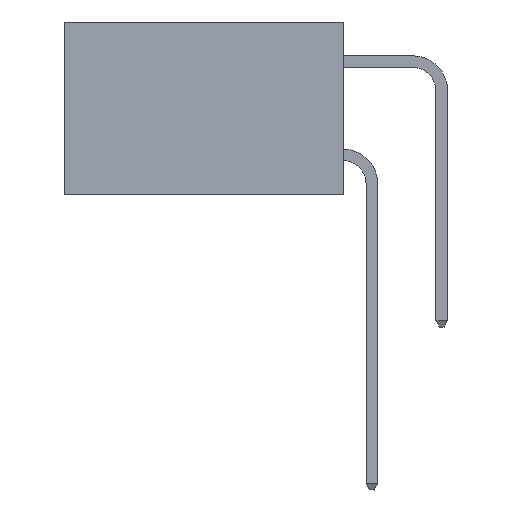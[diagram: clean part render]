
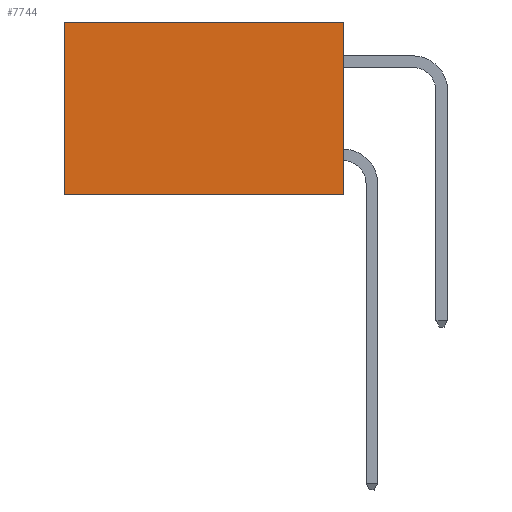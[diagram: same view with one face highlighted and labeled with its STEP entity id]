
A CAD part, left-side view. The second image highlights one B-rep face of the part: STEP entity #7744.
In plain terms, the highlighted planar face has unit normal (-1, 0, 0).
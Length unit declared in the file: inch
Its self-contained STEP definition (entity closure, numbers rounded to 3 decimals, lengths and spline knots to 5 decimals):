
#1168 = DIRECTION ( 'NONE',  ( 0., 1., 0. ) ) ;
#1582 = ORIENTED_EDGE ( 'NONE', *, *, #8854, .F. ) ;
#1912 = DIRECTION ( 'NONE',  ( 0., 0., -1. ) ) ;
#1956 = DIRECTION ( 'NONE',  ( 1., 0., 0. ) ) ;
#1972 = CARTESIAN_POINT ( 'NONE',  ( 0.298, 0., 0. ) ) ;
#2181 = PLANE ( 'NONE',  #12047 ) ;
#4954 = EDGE_CURVE ( 'NONE', #11931, #9346, #11756, .T. ) ;
#5278 = VERTEX_POINT ( 'NONE', #7902 ) ;
#5375 = ORIENTED_EDGE ( 'NONE', *, *, #5429, .T. ) ;
#5429 = EDGE_CURVE ( 'NONE', #9346, #5278, #15580, .T. ) ;
#5762 = EDGE_LOOP ( 'NONE', ( #5375, #16929, #1582, #7177 ) ) ;
#6654 = FACE_OUTER_BOUND ( 'NONE', #5762, .T. ) ;
#7177 = ORIENTED_EDGE ( 'NONE', *, *, #4954, .T. ) ;
#7356 = VECTOR ( 'NONE', #11741, 39.37008 ) ;
#7744 = ADVANCED_FACE ( 'NONE', ( #6654 ), #2181, .F. ) ;
#7902 = CARTESIAN_POINT ( 'NONE',  ( 0.298, 0.6, -0.37 ) ) ;
#8142 = DIRECTION ( 'NONE',  ( 0., 0., -1. ) ) ;
#8854 = EDGE_CURVE ( 'NONE', #11931, #17126, #16769, .T. ) ;
#9346 = VERTEX_POINT ( 'NONE', #12626 ) ;
#9429 = EDGE_CURVE ( 'NONE', #17126, #5278, #10902, .T. ) ;
#10347 = CARTESIAN_POINT ( 'NONE',  ( 0.298, 0.6, 0. ) ) ;
#10902 = LINE ( 'NONE', #11955, #7356 ) ;
#11355 = VECTOR ( 'NONE', #1168, 39.37008 ) ;
#11741 = DIRECTION ( 'NONE',  ( 0., 1., 0. ) ) ;
#11756 = LINE ( 'NONE', #15293, #11355 ) ;
#11931 = VERTEX_POINT ( 'NONE', #13802 ) ;
#11955 = CARTESIAN_POINT ( 'NONE',  ( 0.298, 0., -0.37 ) ) ;
#12047 = AXIS2_PLACEMENT_3D ( 'NONE', #1972, #1956, #1912 ) ;
#12626 = CARTESIAN_POINT ( 'NONE',  ( 0.298, 0.6, 0. ) ) ;
#13070 = CARTESIAN_POINT ( 'NONE',  ( 0.298, 0., -0.37 ) ) ;
#13802 = CARTESIAN_POINT ( 'NONE',  ( 0.298, 0., 0. ) ) ;
#14762 = VECTOR ( 'NONE', #8142, 39.37008 ) ;
#15293 = CARTESIAN_POINT ( 'NONE',  ( 0.298, 0., 0. ) ) ;
#15498 = DIRECTION ( 'NONE',  ( 0., 0., -1. ) ) ;
#15515 = CARTESIAN_POINT ( 'NONE',  ( 0.298, 0., 0. ) ) ;
#15580 = LINE ( 'NONE', #10347, #14762 ) ;
#16366 = VECTOR ( 'NONE', #15498, 39.37008 ) ;
#16769 = LINE ( 'NONE', #15515, #16366 ) ;
#16929 = ORIENTED_EDGE ( 'NONE', *, *, #9429, .F. ) ;
#17126 = VERTEX_POINT ( 'NONE', #13070 ) ;
